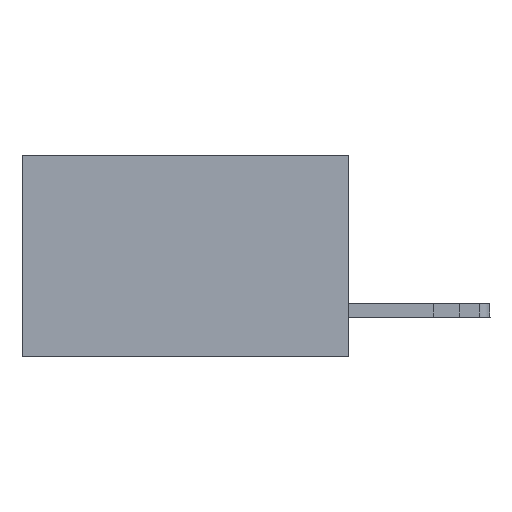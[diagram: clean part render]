
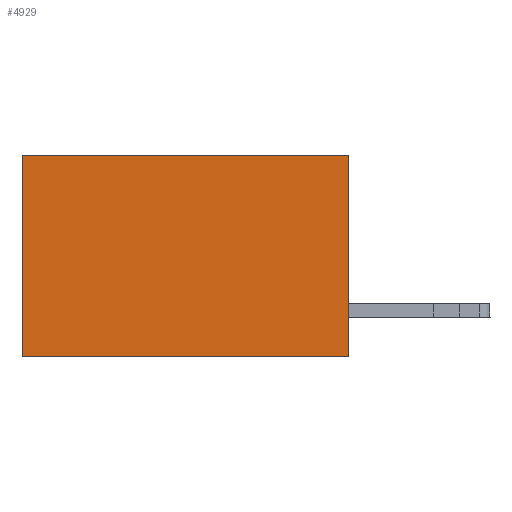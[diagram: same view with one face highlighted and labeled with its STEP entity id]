
A CAD part, left-side view. The second image highlights one B-rep face of the part: STEP entity #4929.
In plain terms, the highlighted planar face has unit normal (-1, 0, 0).
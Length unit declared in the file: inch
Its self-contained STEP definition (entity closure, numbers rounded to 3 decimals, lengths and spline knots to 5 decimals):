
#512 = ORIENTED_EDGE ( 'NONE', *, *, #12936, .F. ) ;
#939 = EDGE_CURVE ( 'NONE', #6855, #8261, #11380, .T. ) ;
#1215 = VECTOR ( 'NONE', #17421, 39.37008 ) ;
#1279 = EDGE_CURVE ( 'NONE', #8261, #9567, #21696, .T. ) ;
#1820 = CARTESIAN_POINT ( 'NONE',  ( 0.298, 0.6, -0.37 ) ) ;
#2371 = CARTESIAN_POINT ( 'NONE',  ( 0.298, 0., -0.37 ) ) ;
#4054 = DIRECTION ( 'NONE',  ( 1., 0., 0. ) ) ;
#4929 = ADVANCED_FACE ( 'NONE', ( #22868 ), #8208, .F. ) ;
#5284 = CARTESIAN_POINT ( 'NONE',  ( 0.298, 0., -0.37 ) ) ;
#6386 = LINE ( 'NONE', #2371, #17843 ) ;
#6855 = VERTEX_POINT ( 'NONE', #10747 ) ;
#7147 = EDGE_CURVE ( 'NONE', #24181, #9567, #6386, .T. ) ;
#7157 = DIRECTION ( 'NONE',  ( 0., 0., -1. ) ) ;
#7727 = EDGE_LOOP ( 'NONE', ( #16214, #9592, #512, #16275 ) ) ;
#8208 = PLANE ( 'NONE',  #22390 ) ;
#8261 = VERTEX_POINT ( 'NONE', #19857 ) ;
#8612 = VECTOR ( 'NONE', #9333, 39.37008 ) ;
#9333 = DIRECTION ( 'NONE',  ( 0., 0., -1. ) ) ;
#9567 = VERTEX_POINT ( 'NONE', #1820 ) ;
#9592 = ORIENTED_EDGE ( 'NONE', *, *, #7147, .F. ) ;
#10627 = CARTESIAN_POINT ( 'NONE',  ( 0.298, 0., 0. ) ) ;
#10747 = CARTESIAN_POINT ( 'NONE',  ( 0.298, 0., 0. ) ) ;
#11380 = LINE ( 'NONE', #13532, #1215 ) ;
#12936 = EDGE_CURVE ( 'NONE', #6855, #24181, #21168, .T. ) ;
#13532 = CARTESIAN_POINT ( 'NONE',  ( 0.298, 0., 0. ) ) ;
#14273 = DIRECTION ( 'NONE',  ( 0., 0., -1. ) ) ;
#16214 = ORIENTED_EDGE ( 'NONE', *, *, #1279, .T. ) ;
#16275 = ORIENTED_EDGE ( 'NONE', *, *, #939, .T. ) ;
#17389 = CARTESIAN_POINT ( 'NONE',  ( 0.298, 0.6, 0. ) ) ;
#17421 = DIRECTION ( 'NONE',  ( 0., 1., 0. ) ) ;
#17843 = VECTOR ( 'NONE', #22814, 39.37008 ) ;
#18006 = VECTOR ( 'NONE', #7157, 39.37008 ) ;
#19857 = CARTESIAN_POINT ( 'NONE',  ( 0.298, 0.6, 0. ) ) ;
#21168 = LINE ( 'NONE', #21570, #8612 ) ;
#21570 = CARTESIAN_POINT ( 'NONE',  ( 0.298, 0., 0. ) ) ;
#21696 = LINE ( 'NONE', #17389, #18006 ) ;
#22390 = AXIS2_PLACEMENT_3D ( 'NONE', #10627, #4054, #14273 ) ;
#22814 = DIRECTION ( 'NONE',  ( 0., 1., 0. ) ) ;
#22868 = FACE_OUTER_BOUND ( 'NONE', #7727, .T. ) ;
#24181 = VERTEX_POINT ( 'NONE', #5284 ) ;
